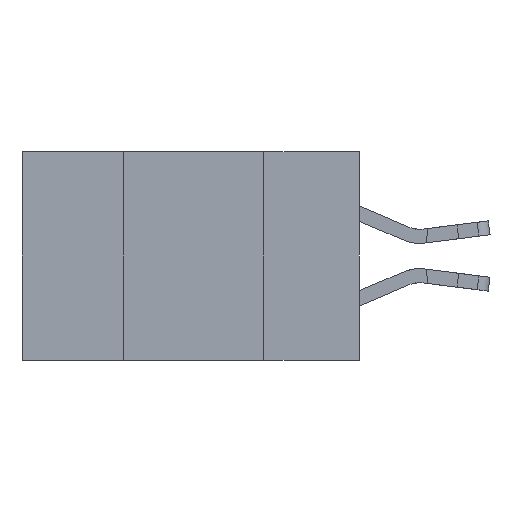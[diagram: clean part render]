
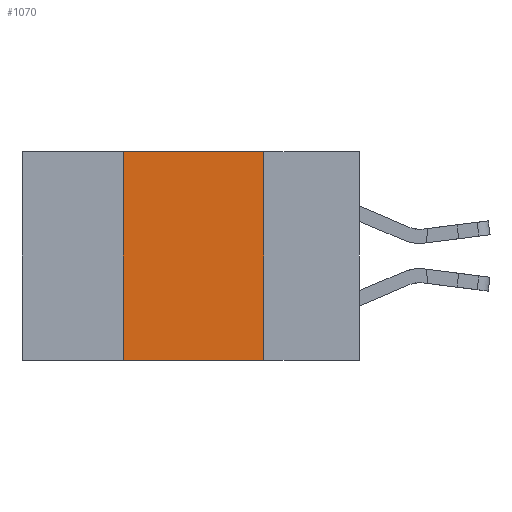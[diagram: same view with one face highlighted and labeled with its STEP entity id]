
A CAD part, left-side view. The second image highlights one B-rep face of the part: STEP entity #1070.
In plain terms, the highlighted planar face has unit normal (-1, 0, 0).
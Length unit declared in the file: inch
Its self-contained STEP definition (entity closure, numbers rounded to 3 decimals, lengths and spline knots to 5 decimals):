
#1070 = ADVANCED_FACE ( 'NONE', ( #13703 ), #17845, .F. ) ;
#1093 = LINE ( 'NONE', #12291, #9562 ) ;
#1255 = AXIS2_PLACEMENT_3D ( 'NONE', #17669, #3896, #6680 ) ;
#2313 = CARTESIAN_POINT ( 'NONE',  ( 0., 0.42, -0.37 ) ) ;
#2483 = ORIENTED_EDGE ( 'NONE', *, *, #17360, .T. ) ;
#2613 = CARTESIAN_POINT ( 'NONE',  ( 0., 0.17, 0. ) ) ;
#2928 = CARTESIAN_POINT ( 'NONE',  ( 0., 0.6, 0. ) ) ;
#3420 = ORIENTED_EDGE ( 'NONE', *, *, #18237, .F. ) ;
#3896 = DIRECTION ( 'NONE',  ( 1., 0., 0. ) ) ;
#4322 = DIRECTION ( 'NONE',  ( 0., 0., 1. ) ) ;
#4909 = EDGE_CURVE ( 'NONE', #7076, #13486, #1093, .T. ) ;
#6676 = VECTOR ( 'NONE', #4322, 39.37008 ) ;
#6680 = DIRECTION ( 'NONE',  ( 0., 0., -1. ) ) ;
#7076 = VERTEX_POINT ( 'NONE', #2613 ) ;
#7088 = DIRECTION ( 'NONE',  ( 0., 0., -1. ) ) ;
#8290 = DIRECTION ( 'NONE',  ( 0., -1., 0. ) ) ;
#8631 = VECTOR ( 'NONE', #8290, 39.37008 ) ;
#8726 = CARTESIAN_POINT ( 'NONE',  ( 0., 0.6, -0.37 ) ) ;
#9298 = VERTEX_POINT ( 'NONE', #11391 ) ;
#9562 = VECTOR ( 'NONE', #7088, 39.37008 ) ;
#10206 = DIRECTION ( 'NONE',  ( 0., -1., 0. ) ) ;
#10297 = ORIENTED_EDGE ( 'NONE', *, *, #13983, .F. ) ;
#11391 = CARTESIAN_POINT ( 'NONE',  ( 0., 0.42, 0. ) ) ;
#12291 = CARTESIAN_POINT ( 'NONE',  ( 0., 0.17, 0. ) ) ;
#12499 = ORIENTED_EDGE ( 'NONE', *, *, #4909, .F. ) ;
#12616 = LINE ( 'NONE', #8726, #18157 ) ;
#12863 = VERTEX_POINT ( 'NONE', #2313 ) ;
#13486 = VERTEX_POINT ( 'NONE', #15317 ) ;
#13703 = FACE_OUTER_BOUND ( 'NONE', #15510, .T. ) ;
#13983 = EDGE_CURVE ( 'NONE', #9298, #7076, #15477, .T. ) ;
#14031 = LINE ( 'NONE', #15496, #6676 ) ;
#15317 = CARTESIAN_POINT ( 'NONE',  ( 0., 0.17, -0.37 ) ) ;
#15477 = LINE ( 'NONE', #2928, #8631 ) ;
#15496 = CARTESIAN_POINT ( 'NONE',  ( 0., 0.42, 0. ) ) ;
#15510 = EDGE_LOOP ( 'NONE', ( #12499, #10297, #3420, #2483 ) ) ;
#17360 = EDGE_CURVE ( 'NONE', #12863, #13486, #12616, .T. ) ;
#17669 = CARTESIAN_POINT ( 'NONE',  ( 0., 0.6, 0. ) ) ;
#17845 = PLANE ( 'NONE',  #1255 ) ;
#18157 = VECTOR ( 'NONE', #10206, 39.37008 ) ;
#18237 = EDGE_CURVE ( 'NONE', #12863, #9298, #14031, .T. ) ;
